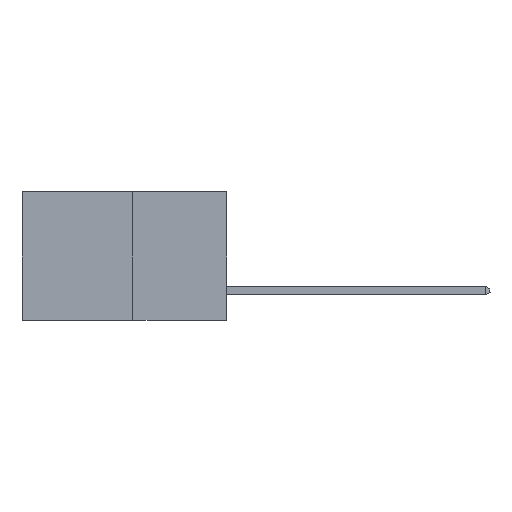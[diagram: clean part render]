
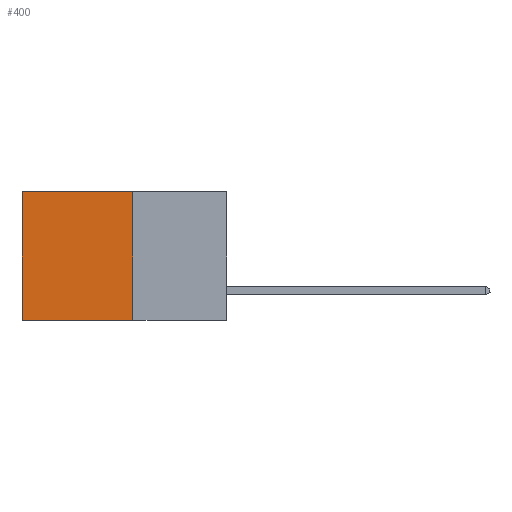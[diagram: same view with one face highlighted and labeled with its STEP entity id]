
A CAD part, left-side view. The second image highlights one B-rep face of the part: STEP entity #400.
In plain terms, the highlighted planar face has unit normal (-1, 0, 0).
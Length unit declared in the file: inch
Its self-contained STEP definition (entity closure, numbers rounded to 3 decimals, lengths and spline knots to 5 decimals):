
#83 = LINE ( 'NONE', #2333, #2539 ) ;
#150 = AXIS2_PLACEMENT_3D ( 'NONE', #2428, #2808, #2794 ) ;
#298 = EDGE_CURVE ( 'NONE', #4706, #5816, #2633, .T. ) ;
#400 = ADVANCED_FACE ( 'NONE', ( #10743 ), #10711, .F. ) ;
#820 = DIRECTION ( 'NONE',  ( 0., 1., 0. ) ) ;
#1396 = ORIENTED_EDGE ( 'NONE', *, *, #13720, .T. ) ;
#1783 = ORIENTED_EDGE ( 'NONE', *, *, #4613, .F. ) ;
#2333 = CARTESIAN_POINT ( 'NONE',  ( 0.277, 0.27, -0.37 ) ) ;
#2428 = CARTESIAN_POINT ( 'NONE',  ( 0.277, 0.27, -0.37 ) ) ;
#2482 = DIRECTION ( 'NONE',  ( 0., 0., -1. ) ) ;
#2517 = ORIENTED_EDGE ( 'NONE', *, *, #6936, .T. ) ;
#2539 = VECTOR ( 'NONE', #3532, 39.37008 ) ;
#2633 = LINE ( 'NONE', #3135, #8117 ) ;
#2794 = DIRECTION ( 'NONE',  ( 0., 0., -1. ) ) ;
#2808 = DIRECTION ( 'NONE',  ( 1., 0., 0. ) ) ;
#3135 = CARTESIAN_POINT ( 'NONE',  ( 0.277, 0.27, -0.37 ) ) ;
#3171 = LINE ( 'NONE', #5889, #11364 ) ;
#3532 = DIRECTION ( 'NONE',  ( 0., 1., 0. ) ) ;
#4613 = EDGE_CURVE ( 'NONE', #5816, #6802, #83, .T. ) ;
#4706 = VERTEX_POINT ( 'NONE', #7914 ) ;
#5649 = VERTEX_POINT ( 'NONE', #5930 ) ;
#5778 = VECTOR ( 'NONE', #820, 39.37008 ) ;
#5816 = VERTEX_POINT ( 'NONE', #10296 ) ;
#5889 = CARTESIAN_POINT ( 'NONE',  ( 0.277, 0.59, -0.37 ) ) ;
#5930 = CARTESIAN_POINT ( 'NONE',  ( 0.277, 0.59, 0. ) ) ;
#6802 = VERTEX_POINT ( 'NONE', #9500 ) ;
#6936 = EDGE_CURVE ( 'NONE', #4706, #5649, #8897, .T. ) ;
#7914 = CARTESIAN_POINT ( 'NONE',  ( 0.277, 0.27, 0. ) ) ;
#8117 = VECTOR ( 'NONE', #13237, 39.37008 ) ;
#8599 = CARTESIAN_POINT ( 'NONE',  ( 0.277, 0.27, 0. ) ) ;
#8897 = LINE ( 'NONE', #8599, #5778 ) ;
#9500 = CARTESIAN_POINT ( 'NONE',  ( 0.277, 0.59, -0.37 ) ) ;
#10296 = CARTESIAN_POINT ( 'NONE',  ( 0.277, 0.27, -0.37 ) ) ;
#10711 = PLANE ( 'NONE',  #150 ) ;
#10743 = FACE_OUTER_BOUND ( 'NONE', #11867, .T. ) ;
#11364 = VECTOR ( 'NONE', #2482, 39.37008 ) ;
#11867 = EDGE_LOOP ( 'NONE', ( #1396, #1783, #13218, #2517 ) ) ;
#13218 = ORIENTED_EDGE ( 'NONE', *, *, #298, .F. ) ;
#13237 = DIRECTION ( 'NONE',  ( 0., 0., -1. ) ) ;
#13720 = EDGE_CURVE ( 'NONE', #5649, #6802, #3171, .T. ) ;
